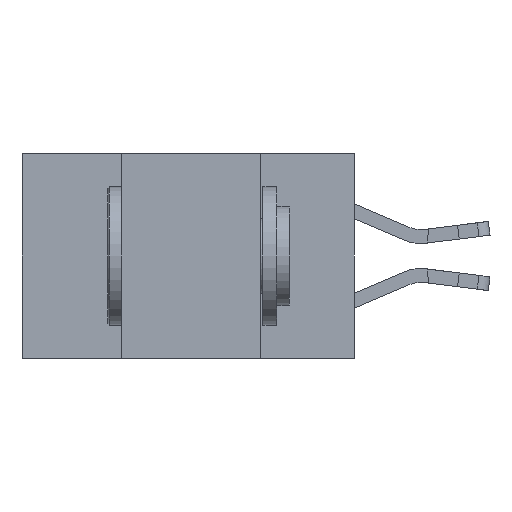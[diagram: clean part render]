
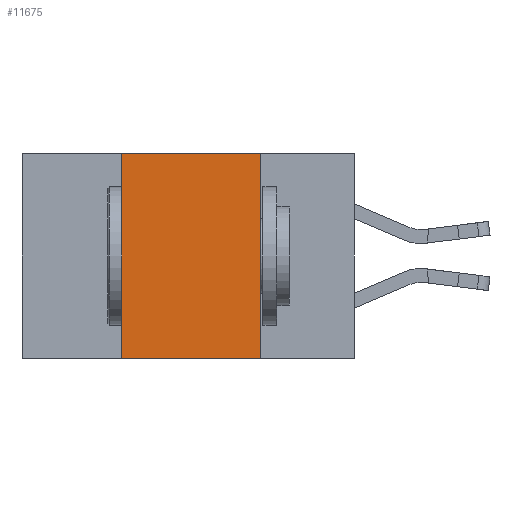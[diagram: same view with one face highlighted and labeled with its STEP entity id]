
A CAD part, left-side view. The second image highlights one B-rep face of the part: STEP entity #11675.
In plain terms, the highlighted planar face has unit normal (-1, 0, 0).
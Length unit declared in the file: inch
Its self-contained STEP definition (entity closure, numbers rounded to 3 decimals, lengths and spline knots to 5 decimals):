
#1557 = LINE ( 'NONE', #16858, #3901 ) ;
#1612 = DIRECTION ( 'NONE',  ( 0., 0., -1. ) ) ;
#3537 = CARTESIAN_POINT ( 'NONE',  ( 0., 0.6, 0. ) ) ;
#3607 = ORIENTED_EDGE ( 'NONE', *, *, #16877, .F. ) ;
#3901 = VECTOR ( 'NONE', #4372, 39.37008 ) ;
#4372 = DIRECTION ( 'NONE',  ( 0., -1., 0. ) ) ;
#5055 = CARTESIAN_POINT ( 'NONE',  ( 0., 0.6, 0. ) ) ;
#5387 = EDGE_CURVE ( 'NONE', #10763, #13039, #1557, .T. ) ;
#5718 = CARTESIAN_POINT ( 'NONE',  ( 0., 0.42, 0. ) ) ;
#6256 = LINE ( 'NONE', #3537, #15454 ) ;
#7518 = EDGE_CURVE ( 'NONE', #17633, #13039, #10030, .T. ) ;
#7613 = DIRECTION ( 'NONE',  ( 0., -1., 0. ) ) ;
#7818 = CARTESIAN_POINT ( 'NONE',  ( 0., 0.42, -0.37 ) ) ;
#9311 = DIRECTION ( 'NONE',  ( 1., 0., 0. ) ) ;
#9403 = PLANE ( 'NONE',  #12286 ) ;
#9695 = VERTEX_POINT ( 'NONE', #5718 ) ;
#9951 = ORIENTED_EDGE ( 'NONE', *, *, #5387, .T. ) ;
#10030 = LINE ( 'NONE', #11118, #15226 ) ;
#10432 = ORIENTED_EDGE ( 'NONE', *, *, #15766, .F. ) ;
#10631 = CARTESIAN_POINT ( 'NONE',  ( 0., 0.17, 0. ) ) ;
#10763 = VERTEX_POINT ( 'NONE', #7818 ) ;
#11118 = CARTESIAN_POINT ( 'NONE',  ( 0., 0.17, -0.37 ) ) ;
#11656 = CARTESIAN_POINT ( 'NONE',  ( 0., 0.17, -0.37 ) ) ;
#11675 = ADVANCED_FACE ( 'NONE', ( #16291 ), #9403, .F. ) ;
#12286 = AXIS2_PLACEMENT_3D ( 'NONE', #5055, #9311, #13288 ) ;
#12332 = DIRECTION ( 'NONE',  ( 0., 0., 1. ) ) ;
#13039 = VERTEX_POINT ( 'NONE', #11656 ) ;
#13288 = DIRECTION ( 'NONE',  ( 0., 0., -1. ) ) ;
#14414 = ORIENTED_EDGE ( 'NONE', *, *, #7518, .F. ) ;
#14660 = EDGE_LOOP ( 'NONE', ( #14414, #10432, #3607, #9951 ) ) ;
#15226 = VECTOR ( 'NONE', #1612, 39.37008 ) ;
#15454 = VECTOR ( 'NONE', #7613, 39.37008 ) ;
#15766 = EDGE_CURVE ( 'NONE', #9695, #17633, #6256, .T. ) ;
#16291 = FACE_OUTER_BOUND ( 'NONE', #14660, .T. ) ;
#16330 = CARTESIAN_POINT ( 'NONE',  ( 0., 0.42, -0.37 ) ) ;
#16858 = CARTESIAN_POINT ( 'NONE',  ( 0., 0.6, -0.37 ) ) ;
#16877 = EDGE_CURVE ( 'NONE', #10763, #9695, #17699, .T. ) ;
#17633 = VERTEX_POINT ( 'NONE', #10631 ) ;
#17699 = LINE ( 'NONE', #16330, #17832 ) ;
#17832 = VECTOR ( 'NONE', #12332, 39.37008 ) ;
